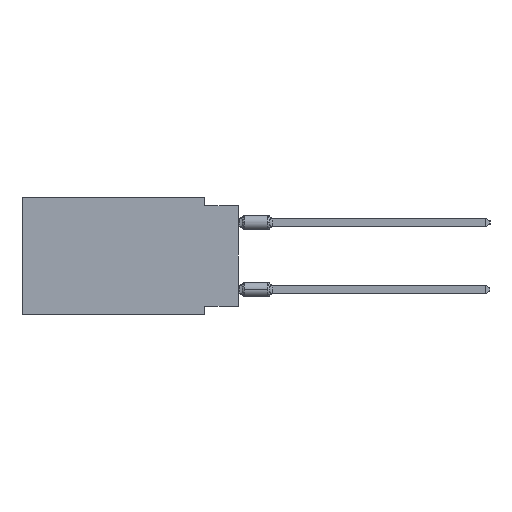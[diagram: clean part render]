
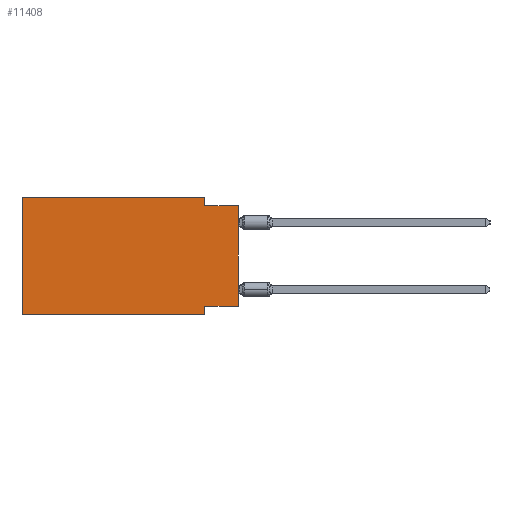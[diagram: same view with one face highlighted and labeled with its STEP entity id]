
A CAD part, left-side view. The second image highlights one B-rep face of the part: STEP entity #11408.
In plain terms, the highlighted planar face has unit normal (-1, 0, 0).
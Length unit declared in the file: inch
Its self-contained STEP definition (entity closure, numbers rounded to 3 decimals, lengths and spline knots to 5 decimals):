
#2847 = DIRECTION ( 'NONE',  ( 0., 0., 1. ) ) ;
#2865 = VECTOR ( 'NONE', #7081, 39.37008 ) ;
#3132 = EDGE_CURVE ( 'NONE', #10732, #26942, #31955, .T. ) ;
#3445 = CARTESIAN_POINT ( 'NONE',  ( 0., 0.645, -0.35 ) ) ;
#4129 = ORIENTED_EDGE ( 'NONE', *, *, #51860, .F. ) ;
#4552 = EDGE_CURVE ( 'NONE', #46209, #16721, #51483, .T. ) ;
#4913 = DIRECTION ( 'NONE',  ( 0., 0., -1. ) ) ;
#5863 = CARTESIAN_POINT ( 'NONE',  ( 0., 0.1, -0.325 ) ) ;
#6221 = AXIS2_PLACEMENT_3D ( 'NONE', #45902, #22764, #4913 ) ;
#6696 = VECTOR ( 'NONE', #12205, 39.37008 ) ;
#7081 = DIRECTION ( 'NONE',  ( 0., 0., 1. ) ) ;
#8284 = DIRECTION ( 'NONE',  ( 0., 0., -1. ) ) ;
#9171 = LINE ( 'NONE', #53080, #26601 ) ;
#10732 = VERTEX_POINT ( 'NONE', #32883 ) ;
#11272 = CARTESIAN_POINT ( 'NONE',  ( 0., 0.645, -0.35 ) ) ;
#11408 = ADVANCED_FACE ( 'NONE', ( #49678 ), #36500, .F. ) ;
#11436 = DIRECTION ( 'NONE',  ( 0., -1., 0. ) ) ;
#12058 = VERTEX_POINT ( 'NONE', #14671 ) ;
#12205 = DIRECTION ( 'NONE',  ( 0., -1., 0. ) ) ;
#12271 = CARTESIAN_POINT ( 'NONE',  ( 0., 0.1, -0.025 ) ) ;
#13231 = CARTESIAN_POINT ( 'NONE',  ( 0., 0., -0.325 ) ) ;
#13789 = ORIENTED_EDGE ( 'NONE', *, *, #47247, .F. ) ;
#14137 = LINE ( 'NONE', #22630, #16421 ) ;
#14671 = CARTESIAN_POINT ( 'NONE',  ( 0., 0., -0.025 ) ) ;
#15573 = CARTESIAN_POINT ( 'NONE',  ( 0., 0., 0. ) ) ;
#16421 = VECTOR ( 'NONE', #8284, 39.37008 ) ;
#16721 = VERTEX_POINT ( 'NONE', #12271 ) ;
#16982 = VECTOR ( 'NONE', #46803, 39.37008 ) ;
#17014 = EDGE_CURVE ( 'NONE', #21537, #43735, #48214, .T. ) ;
#20532 = CARTESIAN_POINT ( 'NONE',  ( 0., 0.1, 0. ) ) ;
#21066 = CARTESIAN_POINT ( 'NONE',  ( 0., 0., -0.025 ) ) ;
#21537 = VERTEX_POINT ( 'NONE', #11272 ) ;
#21732 = CARTESIAN_POINT ( 'NONE',  ( 0., 0.645, 0. ) ) ;
#21930 = VECTOR ( 'NONE', #11436, 39.37008 ) ;
#22630 = CARTESIAN_POINT ( 'NONE',  ( 0., 0.1, -0.35 ) ) ;
#22736 = EDGE_CURVE ( 'NONE', #21537, #38873, #38831, .T. ) ;
#22764 = DIRECTION ( 'NONE',  ( 1., 0., 0. ) ) ;
#24353 = EDGE_CURVE ( 'NONE', #10732, #12058, #25195, .T. ) ;
#25005 = ORIENTED_EDGE ( 'NONE', *, *, #3132, .F. ) ;
#25195 = LINE ( 'NONE', #15573, #2865 ) ;
#25490 = VECTOR ( 'NONE', #36068, 39.37008 ) ;
#25571 = CARTESIAN_POINT ( 'NONE',  ( 0., 0.1, -0.35 ) ) ;
#26601 = VECTOR ( 'NONE', #30812, 39.37008 ) ;
#26942 = VERTEX_POINT ( 'NONE', #5863 ) ;
#29858 = ORIENTED_EDGE ( 'NONE', *, *, #53608, .F. ) ;
#30812 = DIRECTION ( 'NONE',  ( 0., -1., 0. ) ) ;
#31643 = ORIENTED_EDGE ( 'NONE', *, *, #4552, .F. ) ;
#31955 = LINE ( 'NONE', #13231, #25490 ) ;
#32523 = EDGE_LOOP ( 'NONE', ( #39780, #29858, #31643, #4129, #46668, #53479, #13789, #25005 ) ) ;
#32883 = CARTESIAN_POINT ( 'NONE',  ( 0., 0., -0.325 ) ) ;
#36068 = DIRECTION ( 'NONE',  ( 0., 1., 0. ) ) ;
#36500 = PLANE ( 'NONE',  #6221 ) ;
#37745 = CARTESIAN_POINT ( 'NONE',  ( 0., 0.1, 0. ) ) ;
#38831 = LINE ( 'NONE', #43795, #41178 ) ;
#38873 = VERTEX_POINT ( 'NONE', #21732 ) ;
#39780 = ORIENTED_EDGE ( 'NONE', *, *, #24353, .T. ) ;
#41178 = VECTOR ( 'NONE', #2847, 39.37008 ) ;
#43735 = VERTEX_POINT ( 'NONE', #25571 ) ;
#43795 = CARTESIAN_POINT ( 'NONE',  ( 0., 0.645, 0. ) ) ;
#45902 = CARTESIAN_POINT ( 'NONE',  ( 0., 0.645, 0. ) ) ;
#46209 = VERTEX_POINT ( 'NONE', #20532 ) ;
#46668 = ORIENTED_EDGE ( 'NONE', *, *, #22736, .F. ) ;
#46803 = DIRECTION ( 'NONE',  ( 0., 0., -1. ) ) ;
#47247 = EDGE_CURVE ( 'NONE', #26942, #43735, #14137, .T. ) ;
#48214 = LINE ( 'NONE', #3445, #6696 ) ;
#49678 = FACE_OUTER_BOUND ( 'NONE', #32523, .T. ) ;
#51483 = LINE ( 'NONE', #37745, #16982 ) ;
#51860 = EDGE_CURVE ( 'NONE', #38873, #46209, #9171, .T. ) ;
#53080 = CARTESIAN_POINT ( 'NONE',  ( 0., 0.645, 0. ) ) ;
#53472 = LINE ( 'NONE', #21066, #21930 ) ;
#53479 = ORIENTED_EDGE ( 'NONE', *, *, #17014, .T. ) ;
#53608 = EDGE_CURVE ( 'NONE', #16721, #12058, #53472, .T. ) ;
